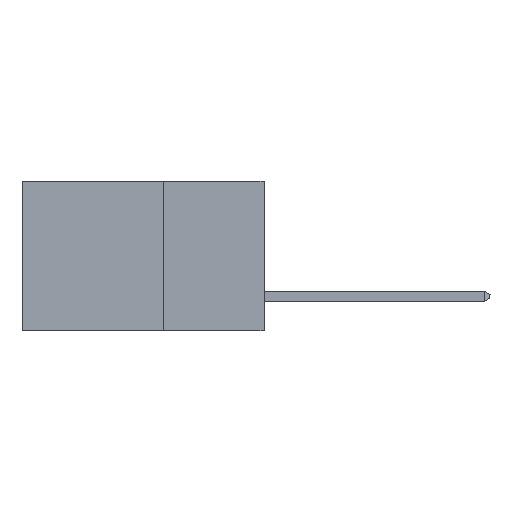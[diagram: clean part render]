
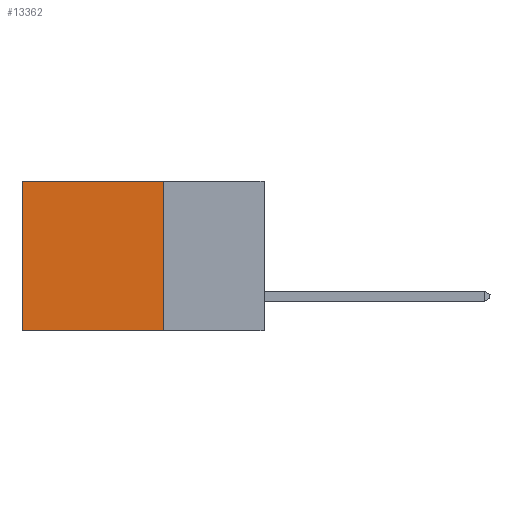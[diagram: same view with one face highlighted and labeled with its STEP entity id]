
A CAD part, left-side view. The second image highlights one B-rep face of the part: STEP entity #13362.
In plain terms, the highlighted planar face has unit normal (-1, 0, 0).
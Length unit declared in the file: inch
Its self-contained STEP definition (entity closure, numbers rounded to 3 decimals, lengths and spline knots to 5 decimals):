
#270 = CARTESIAN_POINT ( 'NONE',  ( 0.2615, 0.6, -0.37 ) ) ;
#690 = DIRECTION ( 'NONE',  ( 1., 0., 0. ) ) ;
#2379 = CARTESIAN_POINT ( 'NONE',  ( 0.2615, 0.25, -0.37 ) ) ;
#2474 = DIRECTION ( 'NONE',  ( 0., 0., -1. ) ) ;
#2534 = VERTEX_POINT ( 'NONE', #270 ) ;
#2636 = LINE ( 'NONE', #13765, #7122 ) ;
#2927 = VECTOR ( 'NONE', #6721, 39.37008 ) ;
#3657 = EDGE_CURVE ( 'NONE', #11863, #10109, #2636, .T. ) ;
#3980 = LINE ( 'NONE', #15231, #3991 ) ;
#3991 = VECTOR ( 'NONE', #15106, 39.37008 ) ;
#5943 = PLANE ( 'NONE',  #13630 ) ;
#6009 = DIRECTION ( 'NONE',  ( 0., 0., -1. ) ) ;
#6721 = DIRECTION ( 'NONE',  ( 0., 1., 0. ) ) ;
#7122 = VECTOR ( 'NONE', #6009, 39.37008 ) ;
#7245 = EDGE_LOOP ( 'NONE', ( #9450, #15108, #15732, #13634 ) ) ;
#9450 = ORIENTED_EDGE ( 'NONE', *, *, #21430, .T. ) ;
#10109 = VERTEX_POINT ( 'NONE', #2379 ) ;
#11566 = EDGE_CURVE ( 'NONE', #10109, #2534, #3980, .T. ) ;
#11863 = VERTEX_POINT ( 'NONE', #18725 ) ;
#12639 = CARTESIAN_POINT ( 'NONE',  ( 0.2615, 0.6, 0. ) ) ;
#13362 = ADVANCED_FACE ( 'NONE', ( #15331 ), #5943, .F. ) ;
#13630 = AXIS2_PLACEMENT_3D ( 'NONE', #22968, #690, #23712 ) ;
#13634 = ORIENTED_EDGE ( 'NONE', *, *, #21152, .T. ) ;
#13765 = CARTESIAN_POINT ( 'NONE',  ( 0.2615, 0.25, -0.37 ) ) ;
#14097 = VECTOR ( 'NONE', #2474, 39.37008 ) ;
#14724 = CARTESIAN_POINT ( 'NONE',  ( 0.2615, 0.25, 0. ) ) ;
#15106 = DIRECTION ( 'NONE',  ( 0., 1., 0. ) ) ;
#15108 = ORIENTED_EDGE ( 'NONE', *, *, #11566, .F. ) ;
#15231 = CARTESIAN_POINT ( 'NONE',  ( 0.2615, 0.25, -0.37 ) ) ;
#15331 = FACE_OUTER_BOUND ( 'NONE', #7245, .T. ) ;
#15732 = ORIENTED_EDGE ( 'NONE', *, *, #3657, .F. ) ;
#18725 = CARTESIAN_POINT ( 'NONE',  ( 0.2615, 0.25, 0. ) ) ;
#19371 = LINE ( 'NONE', #21371, #14097 ) ;
#21152 = EDGE_CURVE ( 'NONE', #11863, #24645, #22490, .T. ) ;
#21371 = CARTESIAN_POINT ( 'NONE',  ( 0.2615, 0.6, -0.37 ) ) ;
#21430 = EDGE_CURVE ( 'NONE', #24645, #2534, #19371, .T. ) ;
#22490 = LINE ( 'NONE', #14724, #2927 ) ;
#22968 = CARTESIAN_POINT ( 'NONE',  ( 0.2615, 0.25, -0.37 ) ) ;
#23712 = DIRECTION ( 'NONE',  ( 0., 0., -1. ) ) ;
#24645 = VERTEX_POINT ( 'NONE', #12639 ) ;
